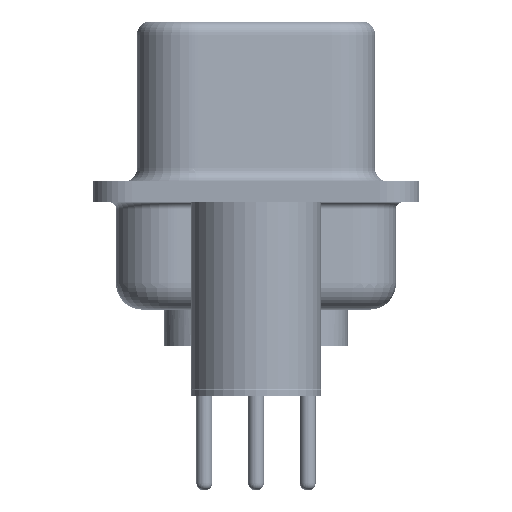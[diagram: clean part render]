
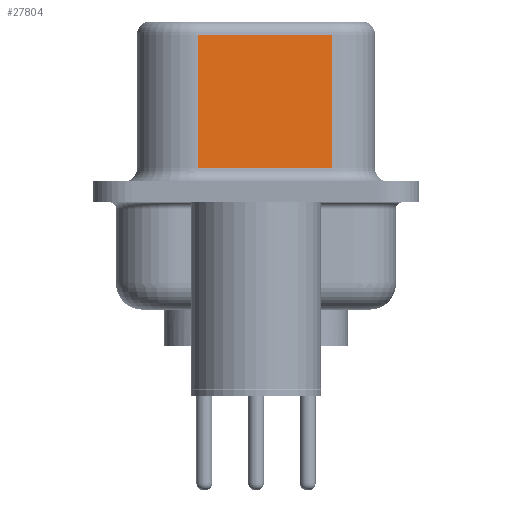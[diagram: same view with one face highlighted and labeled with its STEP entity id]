
A CAD part, left-side view. The second image highlights one B-rep face of the part: STEP entity #27804.
In plain terms, the highlighted planar face has unit normal (-0.985, -0.174, 0).
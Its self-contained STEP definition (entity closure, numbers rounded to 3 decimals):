
#53 = CARTESIAN_POINT ( 'NONE',  ( 3.68, 2.203, 0.9 ) ) ;
#616 = DIRECTION ( 'NONE',  ( 0., 0., -1. ) ) ;
#1582 = CARTESIAN_POINT ( 'NONE',  ( 4.58, -2.897, 6.02 ) ) ;
#1763 = DIRECTION ( 'NONE',  ( 0., 0., -1. ) ) ;
#2225 = EDGE_CURVE ( 'NONE', #3875, #5281, #9131, .T. ) ;
#3875 = VERTEX_POINT ( 'NONE', #32466 ) ;
#4882 = LINE ( 'NONE', #19484, #24481 ) ;
#5281 = VERTEX_POINT ( 'NONE', #53 ) ;
#5361 = VECTOR ( 'NONE', #32887, 1000. ) ;
#5724 = ORIENTED_EDGE ( 'NONE', *, *, #2225, .T. ) ;
#6157 = CARTESIAN_POINT ( 'NONE',  ( 4.58, -2.897, 0.9 ) ) ;
#9131 = LINE ( 'NONE', #18352, #22743 ) ;
#12137 = LINE ( 'NONE', #19883, #24807 ) ;
#15094 = CARTESIAN_POINT ( 'NONE',  ( 4.58, -2.897, 6.52 ) ) ;
#15231 = EDGE_CURVE ( 'NONE', #28368, #3875, #25731, .T. ) ;
#17646 = DIRECTION ( 'NONE',  ( -0.174, 0.985, 0. ) ) ;
#18352 = CARTESIAN_POINT ( 'NONE',  ( 3.68, 2.203, 6.52 ) ) ;
#19484 = CARTESIAN_POINT ( 'NONE',  ( 4.58, -2.897, 0.9 ) ) ;
#19506 = AXIS2_PLACEMENT_3D ( 'NONE', #15094, #32673, #17646 ) ;
#19883 = CARTESIAN_POINT ( 'NONE',  ( 4.58, -2.897, 6.52 ) ) ;
#20483 = ORIENTED_EDGE ( 'NONE', *, *, #30415, .F. ) ;
#22743 = VECTOR ( 'NONE', #616, 1000. ) ;
#24481 = VECTOR ( 'NONE', #29711, 1000. ) ;
#24807 = VECTOR ( 'NONE', #1763, 1000. ) ;
#25292 = FACE_OUTER_BOUND ( 'NONE', #31895, .T. ) ;
#25731 = LINE ( 'NONE', #30402, #5361 ) ;
#26947 = ORIENTED_EDGE ( 'NONE', *, *, #15231, .T. ) ;
#27537 = VERTEX_POINT ( 'NONE', #6157 ) ;
#27804 = ADVANCED_FACE ( 'NONE', ( #25292 ), #30183, .F. ) ;
#28174 = ORIENTED_EDGE ( 'NONE', *, *, #28344, .T. ) ;
#28344 = EDGE_CURVE ( 'NONE', #5281, #27537, #4882, .T. ) ;
#28368 = VERTEX_POINT ( 'NONE', #1582 ) ;
#29711 = DIRECTION ( 'NONE',  ( 0.174, -0.985, 0. ) ) ;
#30183 = PLANE ( 'NONE',  #19506 ) ;
#30402 = CARTESIAN_POINT ( 'NONE',  ( 4.58, -2.897, 6.02 ) ) ;
#30415 = EDGE_CURVE ( 'NONE', #28368, #27537, #12137, .T. ) ;
#31895 = EDGE_LOOP ( 'NONE', ( #20483, #26947, #5724, #28174 ) ) ;
#32466 = CARTESIAN_POINT ( 'NONE',  ( 3.68, 2.203, 6.02 ) ) ;
#32673 = DIRECTION ( 'NONE',  ( 0.985, 0.174, 0. ) ) ;
#32887 = DIRECTION ( 'NONE',  ( -0.174, 0.985, 0. ) ) ;
